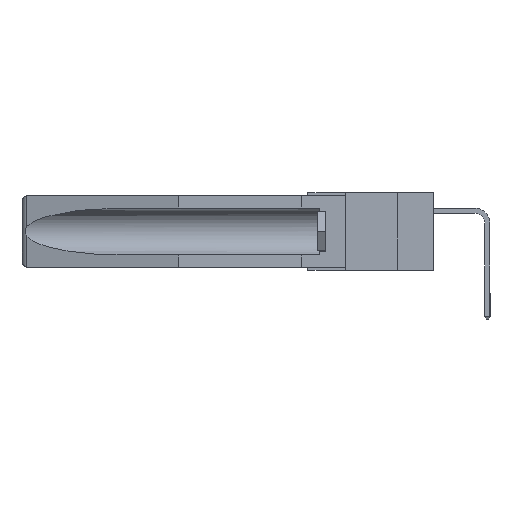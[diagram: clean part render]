
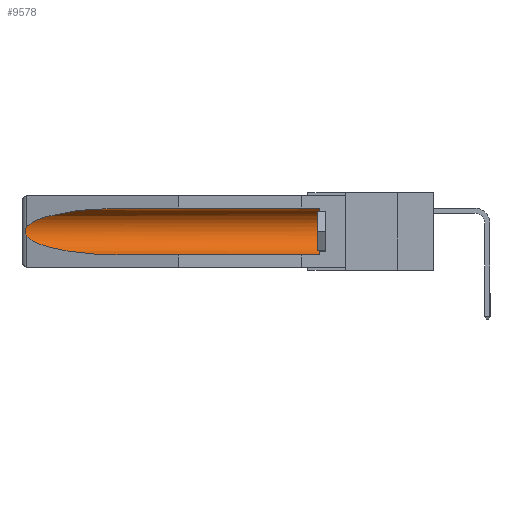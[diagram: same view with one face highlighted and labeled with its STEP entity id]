
A CAD part, left-side view. The second image highlights one B-rep face of the part: STEP entity #9578.
In plain terms, the highlighted cylindrical face has radius 2.857 mm (diameter 5.715 mm), a partial arc.
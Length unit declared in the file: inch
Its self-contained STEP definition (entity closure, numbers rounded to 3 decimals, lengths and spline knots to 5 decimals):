
#25 = VERTEX_POINT ( 'NONE', #9757 ) ;
#450 = CARTESIAN_POINT ( 'NONE',  ( 0.155, 1.07973, -0.059 ) ) ;
#667 = VERTEX_POINT ( 'NONE', #17662 ) ;
#803 = CYLINDRICAL_SURFACE ( 'NONE', #20514, 0.1125 ) ;
#848 = EDGE_CURVE ( 'NONE', #25, #6340, #10320, .T. ) ;
#953 = CARTESIAN_POINT ( 'NONE',  ( 0.2675, 1.53308, -0.17534 ) ) ;
#1668 = EDGE_CURVE ( 'NONE', #25, #14486, #10569, .T. ) ;
#2353 = VECTOR ( 'NONE', #16374, 39.37008 ) ;
#2402 = ORIENTED_EDGE ( 'NONE', *, *, #7781, .T. ) ;
#4270 = ORIENTED_EDGE ( 'NONE', *, *, #5168, .T. ) ;
#4439 = CARTESIAN_POINT ( 'NONE',  ( 0.26655, 1.53094, -0.18657 ) ) ;
#5168 = EDGE_CURVE ( 'NONE', #20805, #10286, #11593, .T. ) ;
#5746 = CARTESIAN_POINT ( 'NONE',  ( 0.155, 0.126, -0.059 ) ) ;
#6021 = CARTESIAN_POINT ( 'NONE',  ( 0.26537, 1.52718, -0.14972 ) ) ;
#6180 = CARTESIAN_POINT ( 'NONE',  ( 0.155, 0.126, -0.1715 ) ) ;
#6328 = CARTESIAN_POINT ( 'NONE',  ( 0.26597, 1.52961, -0.15275 ) ) ;
#6340 = VERTEX_POINT ( 'NONE', #20155 ) ;
#7560 = DIRECTION ( 'NONE',  ( 0., 1., 0. ) ) ;
#7721 =( BOUNDED_CURVE ( )  B_SPLINE_CURVE ( 3, ( #13901, #14055, #20596, #8954 ),
 .UNSPECIFIED., .F., .F. ) 
 B_SPLINE_CURVE_WITH_KNOTS ( ( 4, 4 ),
 ( 0.1948, 1.5708 ),
 .UNSPECIFIED. ) 
 CURVE ( )  GEOMETRIC_REPRESENTATION_ITEM ( )  RATIONAL_B_SPLINE_CURVE ( ( 1., 0.848, 0.848, 1. ) ) 
 REPRESENTATION_ITEM ( '' )  );
#7781 = EDGE_CURVE ( 'NONE', #14486, #667, #11262, .T. ) ;
#7940 = CARTESIAN_POINT ( 'NONE',  ( 0.26537, 1.52718, -0.14972 ) ) ;
#8509 =( BOUNDED_CURVE ( )  B_SPLINE_CURVE ( 3, ( #450, #13829, #14278, #9165 ),
 .UNSPECIFIED., .F., .F. ) 
 B_SPLINE_CURVE_WITH_KNOTS ( ( 4, 4 ),
 ( 4.71239, 6.08839 ),
 .UNSPECIFIED. ) 
 CURVE ( )  GEOMETRIC_REPRESENTATION_ITEM ( )  RATIONAL_B_SPLINE_CURVE ( ( 1., 0.848, 0.848, 1. ) ) 
 REPRESENTATION_ITEM ( '' )  );
#8596 = DIRECTION ( 'NONE',  ( 0., 1., 0. ) ) ;
#8954 = CARTESIAN_POINT ( 'NONE',  ( 0.155, 1.07973, -0.284 ) ) ;
#9165 = CARTESIAN_POINT ( 'NONE',  ( 0.26537, 1.52718, -0.14972 ) ) ;
#9578 = ADVANCED_FACE ( 'NONE', ( #15207 ), #803, .F. ) ;
#9602 = CARTESIAN_POINT ( 'NONE',  ( 0.26654, 1.53092, -0.15636 ) ) ;
#9757 = CARTESIAN_POINT ( 'NONE',  ( 0.155, 0.126, -0.284 ) ) ;
#9802 = CARTESIAN_POINT ( 'NONE',  ( 0.155, -0.30754, -0.059 ) ) ;
#10286 = VERTEX_POINT ( 'NONE', #21057 ) ;
#10320 = LINE ( 'NONE', #16929, #14508 ) ;
#10569 = CIRCLE ( 'NONE', #21508, 0.1125 ) ;
#10894 = DIRECTION ( 'NONE',  ( 0., 0., 1. ) ) ;
#11137 = CARTESIAN_POINT ( 'NONE',  ( 0.26597, 1.5296, -0.19026 ) ) ;
#11167 = EDGE_CURVE ( 'NONE', #10286, #6340, #7721, .T. ) ;
#11262 = LINE ( 'NONE', #9802, #2353 ) ;
#11593 = B_SPLINE_CURVE_WITH_KNOTS ( 'NONE', 3,
 ( #7940, #6328, #9602, #12751, #14408, #953, #16171, #4439, #11137, #17864 ),
 .UNSPECIFIED., .F., .F.,
 ( 4, 2, 2, 2, 4 ),
 ( 0., 0.00029, 0.00058, 0.00087, 0.00117 ),
 .UNSPECIFIED. ) ;
#12751 = CARTESIAN_POINT ( 'NONE',  ( 0.2673, 1.5327, -0.16383 ) ) ;
#13829 = CARTESIAN_POINT ( 'NONE',  ( 0.21114, 1.30732, -0.059 ) ) ;
#13890 = ORIENTED_EDGE ( 'NONE', *, *, #848, .F. ) ;
#13901 = CARTESIAN_POINT ( 'NONE',  ( 0.26537, 1.52718, -0.19328 ) ) ;
#14055 = CARTESIAN_POINT ( 'NONE',  ( 0.25451, 1.48313, -0.24835 ) ) ;
#14278 = CARTESIAN_POINT ( 'NONE',  ( 0.25451, 1.48313, -0.09465 ) ) ;
#14408 = CARTESIAN_POINT ( 'NONE',  ( 0.2675, 1.53308, -0.16763 ) ) ;
#14486 = VERTEX_POINT ( 'NONE', #5746 ) ;
#14508 = VECTOR ( 'NONE', #8596, 39.37008 ) ;
#15103 = ORIENTED_EDGE ( 'NONE', *, *, #18833, .T. ) ;
#15207 = FACE_OUTER_BOUND ( 'NONE', #19928, .T. ) ;
#15791 = CARTESIAN_POINT ( 'NONE',  ( 0.155, -0.30754, -0.1715 ) ) ;
#16171 = CARTESIAN_POINT ( 'NONE',  ( 0.2673, 1.53269, -0.17917 ) ) ;
#16374 = DIRECTION ( 'NONE',  ( 0., 1., 0. ) ) ;
#16929 = CARTESIAN_POINT ( 'NONE',  ( 0.155, -0.30754, -0.284 ) ) ;
#17268 = ORIENTED_EDGE ( 'NONE', *, *, #1668, .T. ) ;
#17662 = CARTESIAN_POINT ( 'NONE',  ( 0.155, 1.07973, -0.059 ) ) ;
#17671 = ORIENTED_EDGE ( 'NONE', *, *, #11167, .T. ) ;
#17864 = CARTESIAN_POINT ( 'NONE',  ( 0.26537, 1.52718, -0.19328 ) ) ;
#18833 = EDGE_CURVE ( 'NONE', #667, #20805, #8509, .T. ) ;
#19510 = DIRECTION ( 'NONE',  ( 0., -1., 0. ) ) ;
#19928 = EDGE_LOOP ( 'NONE', ( #15103, #4270, #17671, #13890, #17268, #2402 ) ) ;
#20155 = CARTESIAN_POINT ( 'NONE',  ( 0.155, 1.07973, -0.284 ) ) ;
#20514 = AXIS2_PLACEMENT_3D ( 'NONE', #15791, #7560, #20816 ) ;
#20596 = CARTESIAN_POINT ( 'NONE',  ( 0.21114, 1.30732, -0.284 ) ) ;
#20805 = VERTEX_POINT ( 'NONE', #6021 ) ;
#20816 = DIRECTION ( 'NONE',  ( 0., 0., 1. ) ) ;
#21057 = CARTESIAN_POINT ( 'NONE',  ( 0.26537, 1.52718, -0.19328 ) ) ;
#21508 = AXIS2_PLACEMENT_3D ( 'NONE', #6180, #19510, #10894 ) ;
